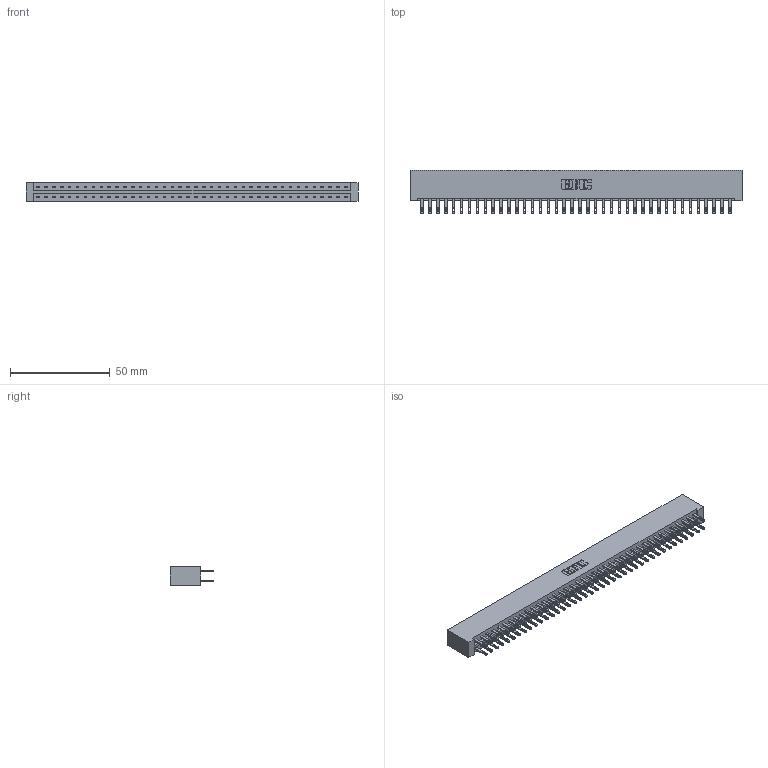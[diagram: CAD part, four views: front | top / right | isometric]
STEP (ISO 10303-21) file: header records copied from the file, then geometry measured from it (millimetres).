
FILE_DESCRIPTION (( 'STEP AP203' ), '1' );
FILE_NAME ('833-080-500-201.STEP', '2020-06-05T21:04:41', ( '' ), ( '' ), 'SwSTEP 2.0', 'SolidWorks 2020', '' );
FILE_SCHEMA (( 'CONFIG_CONTROL_DESIGN' ));
Length unit declared in the file: inch
Products named in the file (3): 345-292-001_345-293-100; 833 Part_Lugless; 833-080-500-201
Assembly tree (81 placements, depth 2):
  833-080-500-201
    833 Part_Lugless
    345-292-001_345-293-100  x80
Bounding box: 166.75 x 21.85 x 9.4 mm (x, y, z)
Volume: 17882.3 mm3; surface area: 22024.6 mm2
Topology: 81 solids, 81 shells, 3946 faces, 12047 edges, 8030 vertices
Faces by surface type: plane 2466, cylinder 1480
Entity records: 25645 total; most frequent: CARTESIAN_POINT 4250, ORIENTED_EDGE 4186, DIRECTION 3629, EDGE_CURVE 2093, LINE 1969, VECTOR 1969, VERTEX_POINT 1394, AXIS2_PLACEMENT_3D 830
